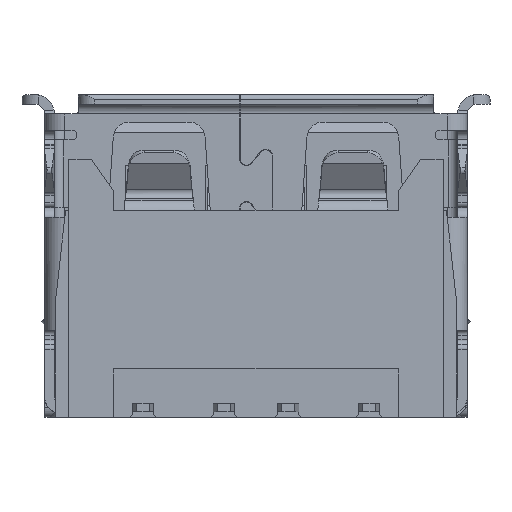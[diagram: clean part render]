
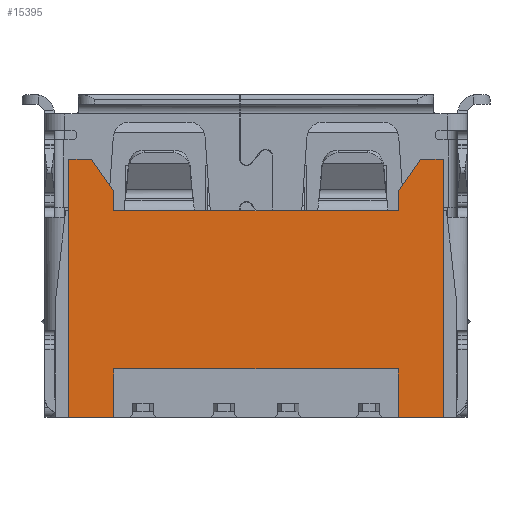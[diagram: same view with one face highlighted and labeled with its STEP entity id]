
A CAD part, front view. The second image highlights one B-rep face of the part: STEP entity #15395.
In plain terms, the highlighted planar face has unit normal (0, -1, 0).
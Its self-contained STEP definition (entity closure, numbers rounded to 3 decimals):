
#446 = VECTOR ( 'NONE', #1069, 1000. ) ;
#745 = DIRECTION ( 'NONE',  ( 1., 0., 0. ) ) ;
#919 = ORIENTED_EDGE ( 'NONE', *, *, #31245, .T. ) ;
#1051 = ORIENTED_EDGE ( 'NONE', *, *, #30111, .T. ) ;
#1069 = DIRECTION ( 'NONE',  ( 0., 0., -1. ) ) ;
#1267 = VECTOR ( 'NONE', #33738, 1000. ) ;
#1287 = CARTESIAN_POINT ( 'NONE',  ( -6.225, -6.65, -1.12 ) ) ;
#1594 = VERTEX_POINT ( 'NONE', #13821 ) ;
#1784 = CARTESIAN_POINT ( 'NONE',  ( 0., -6.65, 6.88 ) ) ;
#1892 = VERTEX_POINT ( 'NONE', #21373 ) ;
#2203 = CARTESIAN_POINT ( 'NONE',  ( -4.4, -6.65, 5.88 ) ) ;
#2683 = VERTEX_POINT ( 'NONE', #18495 ) ;
#2734 = DIRECTION ( 'NONE',  ( 0., 0., 1. ) ) ;
#3249 = VECTOR ( 'NONE', #24071, 1000. ) ;
#3521 = LINE ( 'NONE', #26303, #12680 ) ;
#4309 = LINE ( 'NONE', #5590, #10174 ) ;
#4676 = ORIENTED_EDGE ( 'NONE', *, *, #19880, .T. ) ;
#5220 = ORIENTED_EDGE ( 'NONE', *, *, #30754, .T. ) ;
#5236 = VECTOR ( 'NONE', #31692, 1000. ) ;
#5240 = EDGE_CURVE ( 'NONE', #7352, #13179, #35276, .T. ) ;
#5430 = VECTOR ( 'NONE', #6919, 1000. ) ;
#5590 = CARTESIAN_POINT ( 'NONE',  ( 5.1, -6.65, 6.88 ) ) ;
#5671 = EDGE_CURVE ( 'NONE', #28201, #10419, #34964, .T. ) ;
#5749 = CARTESIAN_POINT ( 'NONE',  ( 4.4, -6.65, 0.38 ) ) ;
#5757 = VECTOR ( 'NONE', #23632, 1000. ) ;
#6055 = EDGE_CURVE ( 'NONE', #31181, #13270, #19829, .T. ) ;
#6919 = DIRECTION ( 'NONE',  ( 0., 0., -1. ) ) ;
#7352 = VERTEX_POINT ( 'NONE', #2203 ) ;
#7563 = CARTESIAN_POINT ( 'NONE',  ( -5.1, -6.65, 6.88 ) ) ;
#7666 = CARTESIAN_POINT ( 'NONE',  ( 5.8, -6.65, 6.88 ) ) ;
#8270 = EDGE_CURVE ( 'NONE', #29576, #33048, #17667, .T. ) ;
#8476 = EDGE_CURVE ( 'NONE', #16874, #28201, #4309, .T. ) ;
#8549 = AXIS2_PLACEMENT_3D ( 'NONE', #20153, #23117, #2734 ) ;
#8551 = EDGE_CURVE ( 'NONE', #1594, #7352, #33560, .T. ) ;
#10019 = CARTESIAN_POINT ( 'NONE',  ( -4.4, -6.65, 0. ) ) ;
#10174 = VECTOR ( 'NONE', #10784, 1000. ) ;
#10419 = VERTEX_POINT ( 'NONE', #20119 ) ;
#10784 = DIRECTION ( 'NONE',  ( -0.573, 0., -0.819 ) ) ;
#10941 = CARTESIAN_POINT ( 'NONE',  ( 0., -6.65, -1.12 ) ) ;
#11283 = FACE_OUTER_BOUND ( 'NONE', #21635, .T. ) ;
#12012 = CARTESIAN_POINT ( 'NONE',  ( 4.4, -6.65, 0. ) ) ;
#12243 = DIRECTION ( 'NONE',  ( -1., 0., 0. ) ) ;
#12495 = ORIENTED_EDGE ( 'NONE', *, *, #8270, .F. ) ;
#12680 = VECTOR ( 'NONE', #12243, 1000. ) ;
#13179 = VERTEX_POINT ( 'NONE', #7563 ) ;
#13263 = LINE ( 'NONE', #20566, #29550 ) ;
#13270 = VERTEX_POINT ( 'NONE', #30833 ) ;
#13821 = CARTESIAN_POINT ( 'NONE',  ( -4.4, -6.65, 5.28 ) ) ;
#14416 = PLANE ( 'NONE',  #8549 ) ;
#14464 = CARTESIAN_POINT ( 'NONE',  ( -5.8, -6.65, 0. ) ) ;
#14984 = VERTEX_POINT ( 'NONE', #5749 ) ;
#15028 = ORIENTED_EDGE ( 'NONE', *, *, #33431, .T. ) ;
#15395 = ADVANCED_FACE ( 'NONE', ( #11283 ), #14416, .T. ) ;
#15557 = CARTESIAN_POINT ( 'NONE',  ( 0., -6.65, 0.38 ) ) ;
#15666 = ORIENTED_EDGE ( 'NONE', *, *, #6055, .T. ) ;
#15913 = ORIENTED_EDGE ( 'NONE', *, *, #5671, .T. ) ;
#16874 = VERTEX_POINT ( 'NONE', #21177 ) ;
#17061 = ORIENTED_EDGE ( 'NONE', *, *, #5240, .T. ) ;
#17667 = LINE ( 'NONE', #34897, #5430 ) ;
#18157 = DIRECTION ( 'NONE',  ( 0., 0., 1. ) ) ;
#18239 = ORIENTED_EDGE ( 'NONE', *, *, #35744, .T. ) ;
#18495 = CARTESIAN_POINT ( 'NONE',  ( -4.4, -6.65, -1.12 ) ) ;
#19660 = VECTOR ( 'NONE', #18157, 1000. ) ;
#19829 = LINE ( 'NONE', #14464, #1267 ) ;
#19847 = CARTESIAN_POINT ( 'NONE',  ( -4.4, -6.65, 0. ) ) ;
#19880 = EDGE_CURVE ( 'NONE', #35882, #33048, #25012, .T. ) ;
#20119 = CARTESIAN_POINT ( 'NONE',  ( 4.4, -6.65, 5.28 ) ) ;
#20153 = CARTESIAN_POINT ( 'NONE',  ( 0., -6.65, 0. ) ) ;
#20397 = VECTOR ( 'NONE', #21594, 1000. ) ;
#20566 = CARTESIAN_POINT ( 'NONE',  ( 4.4, -6.65, 0. ) ) ;
#20591 = LINE ( 'NONE', #26139, #5236 ) ;
#21026 = CARTESIAN_POINT ( 'NONE',  ( -4.4, -6.65, 5.88 ) ) ;
#21120 = LINE ( 'NONE', #10019, #19660 ) ;
#21177 = CARTESIAN_POINT ( 'NONE',  ( 5.1, -6.65, 6.88 ) ) ;
#21373 = CARTESIAN_POINT ( 'NONE',  ( -4.4, -6.65, 0.38 ) ) ;
#21594 = DIRECTION ( 'NONE',  ( -1., 0., 0. ) ) ;
#21635 = EDGE_LOOP ( 'NONE', ( #21787, #15913, #32309, #31402, #17061, #29485, #15666, #1051, #18239, #919, #15028, #4676, #12495, #5220 ) ) ;
#21787 = ORIENTED_EDGE ( 'NONE', *, *, #8476, .T. ) ;
#22401 = EDGE_CURVE ( 'NONE', #10419, #1594, #20591, .T. ) ;
#23117 = DIRECTION ( 'NONE',  ( 0., -1., 0. ) ) ;
#23632 = DIRECTION ( 'NONE',  ( -0.573, 0., 0.819 ) ) ;
#24071 = DIRECTION ( 'NONE',  ( 1., 0., 0. ) ) ;
#24286 = CARTESIAN_POINT ( 'NONE',  ( 5.8, -6.65, -1.12 ) ) ;
#24550 = DIRECTION ( 'NONE',  ( 0., 0., -1. ) ) ;
#25012 = LINE ( 'NONE', #10941, #28824 ) ;
#25592 = DIRECTION ( 'NONE',  ( 0., 0., 1. ) ) ;
#26139 = CARTESIAN_POINT ( 'NONE',  ( 0., -6.65, 5.28 ) ) ;
#26303 = CARTESIAN_POINT ( 'NONE',  ( 0., -6.65, 6.88 ) ) ;
#27181 = LINE ( 'NONE', #1784, #20397 ) ;
#28201 = VERTEX_POINT ( 'NONE', #35814 ) ;
#28824 = VECTOR ( 'NONE', #33352, 1000. ) ;
#29045 = CARTESIAN_POINT ( 'NONE',  ( 4.4, -6.65, -1.12 ) ) ;
#29095 = VECTOR ( 'NONE', #25592, 1000. ) ;
#29485 = ORIENTED_EDGE ( 'NONE', *, *, #30217, .T. ) ;
#29550 = VECTOR ( 'NONE', #24550, 1000. ) ;
#29576 = VERTEX_POINT ( 'NONE', #7666 ) ;
#29622 = LINE ( 'NONE', #1287, #30411 ) ;
#30111 = EDGE_CURVE ( 'NONE', #13270, #2683, #29622, .T. ) ;
#30217 = EDGE_CURVE ( 'NONE', #13179, #31181, #3521, .T. ) ;
#30411 = VECTOR ( 'NONE', #745, 1000. ) ;
#30754 = EDGE_CURVE ( 'NONE', #29576, #16874, #27181, .T. ) ;
#30833 = CARTESIAN_POINT ( 'NONE',  ( -5.8, -6.65, -1.12 ) ) ;
#31181 = VERTEX_POINT ( 'NONE', #34093 ) ;
#31245 = EDGE_CURVE ( 'NONE', #1892, #14984, #31877, .T. ) ;
#31402 = ORIENTED_EDGE ( 'NONE', *, *, #8551, .T. ) ;
#31692 = DIRECTION ( 'NONE',  ( -1., 0., 0. ) ) ;
#31877 = LINE ( 'NONE', #15557, #3249 ) ;
#32309 = ORIENTED_EDGE ( 'NONE', *, *, #22401, .T. ) ;
#33048 = VERTEX_POINT ( 'NONE', #24286 ) ;
#33352 = DIRECTION ( 'NONE',  ( 1., 0., 0. ) ) ;
#33431 = EDGE_CURVE ( 'NONE', #14984, #35882, #13263, .T. ) ;
#33560 = LINE ( 'NONE', #19847, #29095 ) ;
#33738 = DIRECTION ( 'NONE',  ( 0., 0., -1. ) ) ;
#34093 = CARTESIAN_POINT ( 'NONE',  ( -5.8, -6.65, 6.88 ) ) ;
#34897 = CARTESIAN_POINT ( 'NONE',  ( 5.8, -6.65, -2.748 ) ) ;
#34964 = LINE ( 'NONE', #12012, #446 ) ;
#35276 = LINE ( 'NONE', #21026, #5757 ) ;
#35744 = EDGE_CURVE ( 'NONE', #2683, #1892, #21120, .T. ) ;
#35814 = CARTESIAN_POINT ( 'NONE',  ( 4.4, -6.65, 5.88 ) ) ;
#35882 = VERTEX_POINT ( 'NONE', #29045 ) ;
